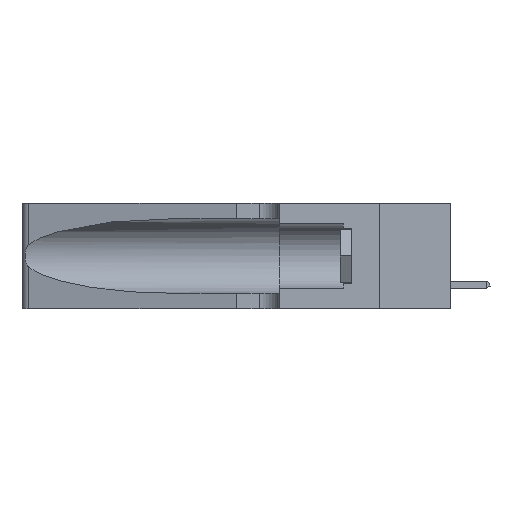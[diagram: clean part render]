
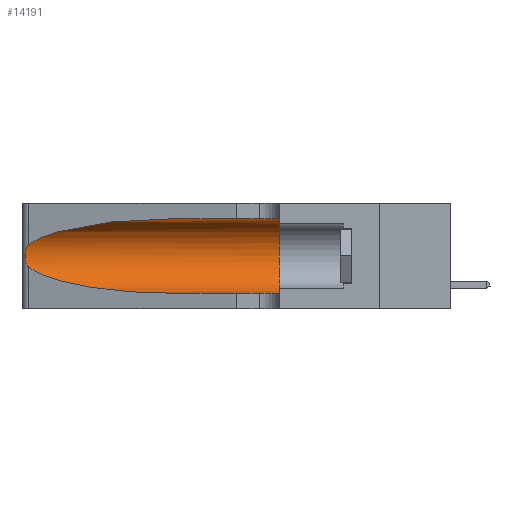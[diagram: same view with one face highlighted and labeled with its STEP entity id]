
A CAD part, left-side view. The second image highlights one B-rep face of the part: STEP entity #14191.
In plain terms, the highlighted cylindrical face has radius 3.308 mm (diameter 6.617 mm), a partial arc.
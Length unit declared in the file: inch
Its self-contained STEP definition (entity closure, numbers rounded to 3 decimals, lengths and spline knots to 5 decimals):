
#85 = ORIENTED_EDGE ( 'NONE', *, *, #10144, .F. ) ;
#532 = VERTEX_POINT ( 'NONE', #11638 ) ;
#616 = CARTESIAN_POINT ( 'NONE',  ( 0.26075, 1.23896, 0.178 ) ) ;
#678 = CARTESIAN_POINT ( 'NONE',  ( 0.25487, 1.22718, 0.14631 ) ) ;
#1008 = LINE ( 'NONE', #3215, #5457 ) ;
#1040 = CARTESIAN_POINT ( 'NONE',  ( 0.1305, 0.72297, 0.05475 ) ) ;
#1298 = VERTEX_POINT ( 'NONE', #1040 ) ;
#1440 = DIRECTION ( 'NONE',  ( 0., 0., 1. ) ) ;
#1939 = CARTESIAN_POINT ( 'NONE',  ( 0.25639, 1.23184, 0.21858 ) ) ;
#1999 = CARTESIAN_POINT ( 'NONE',  ( 0.26075, 1.23896, 0.19203 ) ) ;
#2060 = CARTESIAN_POINT ( 'NONE',  ( 0.25856, 1.23593, 0.16098 ) ) ;
#2583 = EDGE_CURVE ( 'NONE', #2803, #17222, #11030, .T. ) ;
#2803 = VERTEX_POINT ( 'NONE', #11930 ) ;
#2947 = ORIENTED_EDGE ( 'NONE', *, *, #7452, .T. ) ;
#3080 = CARTESIAN_POINT ( 'NONE',  ( 0.1305, 0.35, 0.31525 ) ) ;
#3141 = VERTEX_POINT ( 'NONE', #11759 ) ;
#3215 = CARTESIAN_POINT ( 'NONE',  ( 0.1305, 1.61858, 0.05475 ) ) ;
#3333 = ORIENTED_EDGE ( 'NONE', *, *, #13039, .T. ) ;
#4189 = CARTESIAN_POINT ( 'NONE',  ( 0.18966, 0.96281, 0.31525 ) ) ;
#5457 = VECTOR ( 'NONE', #13103, 39.37008 ) ;
#6017 = VERTEX_POINT ( 'NONE', #8686 ) ;
#6154 =( BOUNDED_CURVE ( )  B_SPLINE_CURVE ( 3, ( #15131, #4189, #9890, #10867 ),
 .UNSPECIFIED., .F., .F. ) 
 B_SPLINE_CURVE_WITH_KNOTS ( ( 4, 4 ),
 ( 1.5708, 2.84003 ),
 .UNSPECIFIED. ) 
 CURVE ( )  GEOMETRIC_REPRESENTATION_ITEM ( )  RATIONAL_B_SPLINE_CURVE ( ( 1., 0.87, 0.87, 1. ) ) 
 REPRESENTATION_ITEM ( '' )  );
#6368 = VECTOR ( 'NONE', #14036, 39.37008 ) ;
#6382 = CARTESIAN_POINT ( 'NONE',  ( 0.25854, 1.2359, 0.20912 ) ) ;
#6619 = CARTESIAN_POINT ( 'NONE',  ( 0.1305, 1.61858, 0.185 ) ) ;
#7055 = ORIENTED_EDGE ( 'NONE', *, *, #2583, .F. ) ;
#7282 = B_SPLINE_CURVE_WITH_KNOTS ( 'NONE', 3,
 ( #17699, #7691, #1939, #13260, #6382, #10661, #1999, #616, #11902, #2060, #13322, #10551, #7747, #678 ),
 .UNSPECIFIED., .F., .F.,
 ( 4, 2, 2, 2, 2, 2, 4 ),
 ( 0., 0.00027, 0.00053, 0.00107, 0.0016, 0.00187, 0.00214 ),
 .UNSPECIFIED. ) ;
#7452 = EDGE_CURVE ( 'NONE', #2803, #532, #6154, .T. ) ;
#7691 = CARTESIAN_POINT ( 'NONE',  ( 0.25555, 1.22994, 0.2215 ) ) ;
#7747 = CARTESIAN_POINT ( 'NONE',  ( 0.25555, 1.22993, 0.14849 ) ) ;
#8041 = DIRECTION ( 'NONE',  ( 0., -1., 0. ) ) ;
#8584 = CIRCLE ( 'NONE', #13059, 0.13025 ) ;
#8686 = CARTESIAN_POINT ( 'NONE',  ( 0.25487, 1.22718, 0.14631 ) ) ;
#8746 = FACE_OUTER_BOUND ( 'NONE', #17104, .T. ) ;
#8954 = CYLINDRICAL_SURFACE ( 'NONE', #14748, 0.13025 ) ;
#9890 = CARTESIAN_POINT ( 'NONE',  ( 0.2373, 1.15595, 0.28018 ) ) ;
#9906 = CARTESIAN_POINT ( 'NONE',  ( 0.1305, 1.61858, 0.31525 ) ) ;
#10144 = EDGE_CURVE ( 'NONE', #17222, #3141, #8584, .T. ) ;
#10551 = CARTESIAN_POINT ( 'NONE',  ( 0.25639, 1.23186, 0.15144 ) ) ;
#10661 = CARTESIAN_POINT ( 'NONE',  ( 0.26018, 1.23835, 0.19895 ) ) ;
#10867 = CARTESIAN_POINT ( 'NONE',  ( 0.25487, 1.22718, 0.22369 ) ) ;
#11030 = LINE ( 'NONE', #9906, #6368 ) ;
#11198 = DIRECTION ( 'NONE',  ( 0., 0., -1. ) ) ;
#11638 = CARTESIAN_POINT ( 'NONE',  ( 0.25487, 1.22718, 0.22369 ) ) ;
#11759 = CARTESIAN_POINT ( 'NONE',  ( 0.1305, 0.35, 0.05475 ) ) ;
#11902 = CARTESIAN_POINT ( 'NONE',  ( 0.26017, 1.23833, 0.17102 ) ) ;
#11930 = CARTESIAN_POINT ( 'NONE',  ( 0.1305, 0.72297, 0.31525 ) ) ;
#12079 = CARTESIAN_POINT ( 'NONE',  ( 0.18966, 0.96281, 0.05475 ) ) ;
#12313 = CARTESIAN_POINT ( 'NONE',  ( 0.2373, 1.15595, 0.08982 ) ) ;
#12817 = ORIENTED_EDGE ( 'NONE', *, *, #18072, .T. ) ;
#13039 = EDGE_CURVE ( 'NONE', #6017, #1298, #15793, .T. ) ;
#13059 = AXIS2_PLACEMENT_3D ( 'NONE', #15421, #14116, #1440 ) ;
#13103 = DIRECTION ( 'NONE',  ( 0., -1., 0. ) ) ;
#13260 = CARTESIAN_POINT ( 'NONE',  ( 0.25787, 1.23484, 0.2124 ) ) ;
#13322 = CARTESIAN_POINT ( 'NONE',  ( 0.25789, 1.23486, 0.15765 ) ) ;
#13440 = CARTESIAN_POINT ( 'NONE',  ( 0.1305, 0.72297, 0.05475 ) ) ;
#14036 = DIRECTION ( 'NONE',  ( 0., -1., 0. ) ) ;
#14116 = DIRECTION ( 'NONE',  ( 0., 1., 0. ) ) ;
#14191 = ADVANCED_FACE ( 'NONE', ( #8746 ), #8954, .F. ) ;
#14748 = AXIS2_PLACEMENT_3D ( 'NONE', #6619, #8041, #11198 ) ;
#15131 = CARTESIAN_POINT ( 'NONE',  ( 0.1305, 0.72297, 0.31525 ) ) ;
#15421 = CARTESIAN_POINT ( 'NONE',  ( 0.1305, 0.35, 0.185 ) ) ;
#15462 = ORIENTED_EDGE ( 'NONE', *, *, #17268, .T. ) ;
#15793 =( BOUNDED_CURVE ( )  B_SPLINE_CURVE ( 3, ( #16481, #12313, #12079, #13440 ),
 .UNSPECIFIED., .F., .F. ) 
 B_SPLINE_CURVE_WITH_KNOTS ( ( 4, 4 ),
 ( 3.44316, 4.71239 ),
 .UNSPECIFIED. ) 
 CURVE ( )  GEOMETRIC_REPRESENTATION_ITEM ( )  RATIONAL_B_SPLINE_CURVE ( ( 1., 0.87, 0.87, 1. ) ) 
 REPRESENTATION_ITEM ( '' )  );
#16481 = CARTESIAN_POINT ( 'NONE',  ( 0.25487, 1.22718, 0.14631 ) ) ;
#17104 = EDGE_LOOP ( 'NONE', ( #2947, #12817, #3333, #15462, #85, #7055 ) ) ;
#17222 = VERTEX_POINT ( 'NONE', #3080 ) ;
#17268 = EDGE_CURVE ( 'NONE', #1298, #3141, #1008, .T. ) ;
#17699 = CARTESIAN_POINT ( 'NONE',  ( 0.25487, 1.22718, 0.22369 ) ) ;
#18072 = EDGE_CURVE ( 'NONE', #532, #6017, #7282, .T. ) ;
